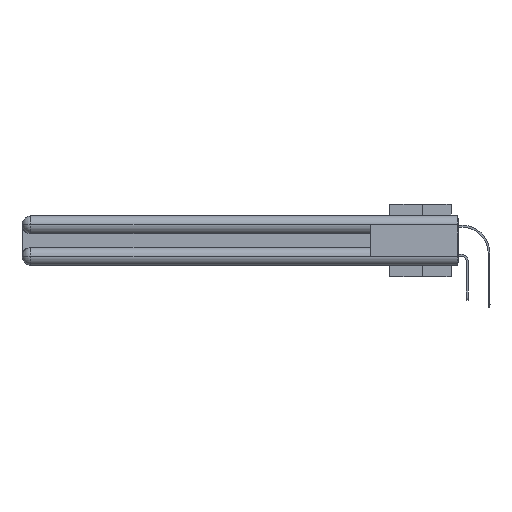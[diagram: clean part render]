
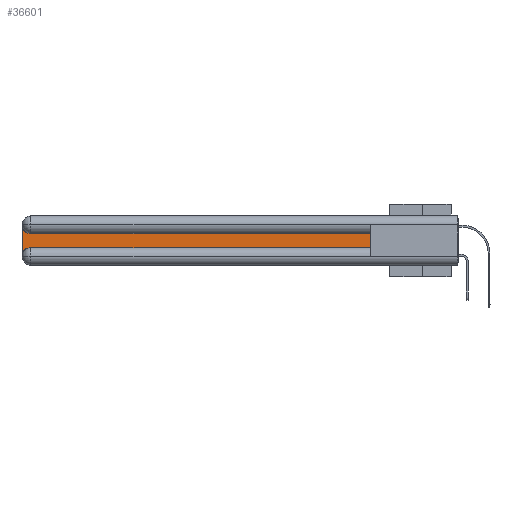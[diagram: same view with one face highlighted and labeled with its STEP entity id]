
A CAD part, left-side view. The second image highlights one B-rep face of the part: STEP entity #36601.
In plain terms, the highlighted planar face has unit normal (-1, 0, 0).
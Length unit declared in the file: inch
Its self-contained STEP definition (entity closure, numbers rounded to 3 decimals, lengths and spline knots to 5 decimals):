
#293 = DIRECTION ( 'NONE',  ( 1., 0., 0. ) ) ;
#1226 = CIRCLE ( 'NONE', #41468, 0.06 ) ;
#2457 = CARTESIAN_POINT ( 'NONE',  ( 0.075, 2.94, -0.2775 ) ) ;
#2785 = DIRECTION ( 'NONE',  ( 1., 0., 0. ) ) ;
#3427 = CARTESIAN_POINT ( 'NONE',  ( 0.075, 3., -0.2775 ) ) ;
#6096 = CARTESIAN_POINT ( 'NONE',  ( 0.075, 0.6, -0.1225 ) ) ;
#8743 = ORIENTED_EDGE ( 'NONE', *, *, #23908, .T. ) ;
#9518 = DIRECTION ( 'NONE',  ( 1., 0., 0. ) ) ;
#10502 = CARTESIAN_POINT ( 'NONE',  ( 0.075, 3., -0.0625 ) ) ;
#10753 = DIRECTION ( 'NONE',  ( 0., -1., 0. ) ) ;
#12303 = DIRECTION ( 'NONE',  ( 0., 0., -1. ) ) ;
#12341 = DIRECTION ( 'NONE',  ( 0., 0., 1. ) ) ;
#12897 = EDGE_CURVE ( 'NONE', #41303, #25239, #15616, .T. ) ;
#13255 = DIRECTION ( 'NONE',  ( 0., 0., -1. ) ) ;
#13556 = LINE ( 'NONE', #16746, #24587 ) ;
#14506 = AXIS2_PLACEMENT_3D ( 'NONE', #35062, #2785, #13255 ) ;
#15090 = ORIENTED_EDGE ( 'NONE', *, *, #34416, .T. ) ;
#15616 = LINE ( 'NONE', #41388, #26668 ) ;
#16462 = PLANE ( 'NONE',  #14506 ) ;
#16505 = CARTESIAN_POINT ( 'NONE',  ( 0.075, 2.94, -0.1225 ) ) ;
#16746 = CARTESIAN_POINT ( 'NONE',  ( 0.075, 0.6, -0.2175 ) ) ;
#16830 = ORIENTED_EDGE ( 'NONE', *, *, #20432, .T. ) ;
#17476 = ORIENTED_EDGE ( 'NONE', *, *, #37633, .T. ) ;
#19014 = FACE_OUTER_BOUND ( 'NONE', #23906, .T. ) ;
#20432 = EDGE_CURVE ( 'NONE', #25239, #41700, #33675, .T. ) ;
#21169 = AXIS2_PLACEMENT_3D ( 'NONE', #32168, #293, #26391 ) ;
#22301 = VECTOR ( 'NONE', #26625, 39.37008 ) ;
#23627 = CARTESIAN_POINT ( 'NONE',  ( 0.075, 2.94, -0.2175 ) ) ;
#23906 = EDGE_LOOP ( 'NONE', ( #16830, #15090, #17476, #8743, #29290, #30869 ) ) ;
#23908 = EDGE_CURVE ( 'NONE', #30232, #38086, #1226, .T. ) ;
#24587 = VECTOR ( 'NONE', #10753, 39.37008 ) ;
#25239 = VERTEX_POINT ( 'NONE', #6096 ) ;
#26391 = DIRECTION ( 'NONE',  ( 0., 0., -1. ) ) ;
#26625 = DIRECTION ( 'NONE',  ( 0., 0., -1. ) ) ;
#26668 = VECTOR ( 'NONE', #12341, 39.37008 ) ;
#26763 = CIRCLE ( 'NONE', #21169, 0.06 ) ;
#27285 = DIRECTION ( 'NONE',  ( 0., 1., 0. ) ) ;
#27798 = EDGE_CURVE ( 'NONE', #38086, #41303, #13556, .T. ) ;
#29290 = ORIENTED_EDGE ( 'NONE', *, *, #27798, .T. ) ;
#29462 = CARTESIAN_POINT ( 'NONE',  ( 0.075, 0.6, -0.2175 ) ) ;
#29789 = VECTOR ( 'NONE', #27285, 39.37008 ) ;
#30232 = VERTEX_POINT ( 'NONE', #3427 ) ;
#30869 = ORIENTED_EDGE ( 'NONE', *, *, #12897, .T. ) ;
#32168 = CARTESIAN_POINT ( 'NONE',  ( 0.075, 2.94, -0.0625 ) ) ;
#33675 = LINE ( 'NONE', #36671, #29789 ) ;
#33684 = VERTEX_POINT ( 'NONE', #10502 ) ;
#34416 = EDGE_CURVE ( 'NONE', #41700, #33684, #26763, .T. ) ;
#35062 = CARTESIAN_POINT ( 'NONE',  ( 0.075, 3., -0.1225 ) ) ;
#36601 = ADVANCED_FACE ( 'NONE', ( #19014 ), #16462, .F. ) ;
#36671 = CARTESIAN_POINT ( 'NONE',  ( 0.075, 0.6, -0.1225 ) ) ;
#37633 = EDGE_CURVE ( 'NONE', #33684, #30232, #39645, .T. ) ;
#38086 = VERTEX_POINT ( 'NONE', #23627 ) ;
#39645 = LINE ( 'NONE', #39850, #22301 ) ;
#39850 = CARTESIAN_POINT ( 'NONE',  ( 0.075, 3., -0.2175 ) ) ;
#41303 = VERTEX_POINT ( 'NONE', #29462 ) ;
#41388 = CARTESIAN_POINT ( 'NONE',  ( 0.075, 0.6, -0.2175 ) ) ;
#41468 = AXIS2_PLACEMENT_3D ( 'NONE', #2457, #9518, #12303 ) ;
#41700 = VERTEX_POINT ( 'NONE', #16505 ) ;
